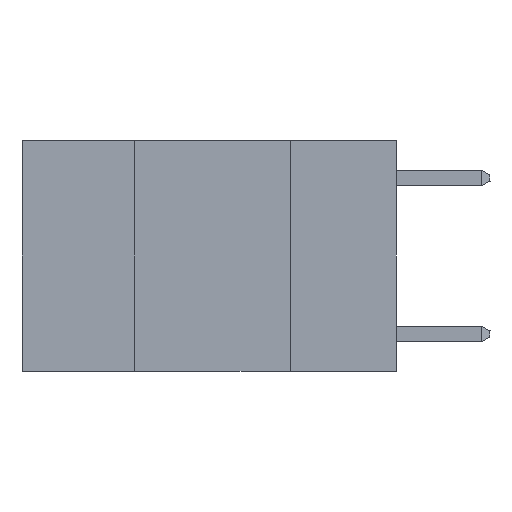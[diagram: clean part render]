
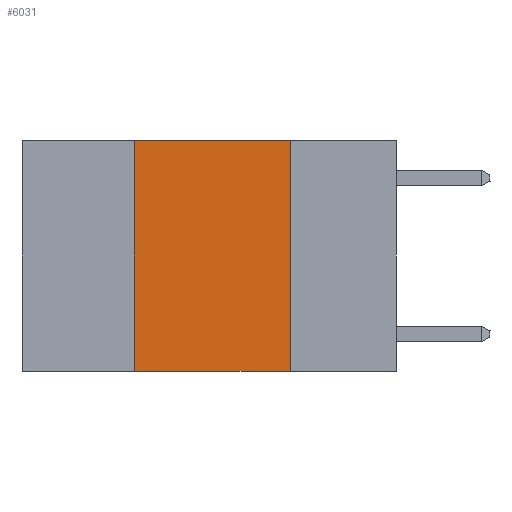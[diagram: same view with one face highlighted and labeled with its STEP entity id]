
A CAD part, left-side view. The second image highlights one B-rep face of the part: STEP entity #6031.
In plain terms, the highlighted planar face has unit normal (-1, 0, 0).
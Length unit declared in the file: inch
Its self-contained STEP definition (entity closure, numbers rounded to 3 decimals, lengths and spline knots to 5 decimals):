
#147 = CARTESIAN_POINT ( 'NONE',  ( 0., 0.6, -0.37 ) ) ;
#323 = LINE ( 'NONE', #3160, #899 ) ;
#630 = VERTEX_POINT ( 'NONE', #1044 ) ;
#771 = VECTOR ( 'NONE', #7086, 39.37008 ) ;
#899 = VECTOR ( 'NONE', #1108, 39.37008 ) ;
#1044 = CARTESIAN_POINT ( 'NONE',  ( 0., 0.17, 0. ) ) ;
#1108 = DIRECTION ( 'NONE',  ( 0., 0., -1. ) ) ;
#1188 = DIRECTION ( 'NONE',  ( 0., 0., -1. ) ) ;
#1454 = CARTESIAN_POINT ( 'NONE',  ( 0., 0.6, 0. ) ) ;
#2038 = LINE ( 'NONE', #6036, #10308 ) ;
#2287 = DIRECTION ( 'NONE',  ( 0., -1., 0. ) ) ;
#2328 = VERTEX_POINT ( 'NONE', #8885 ) ;
#3160 = CARTESIAN_POINT ( 'NONE',  ( 0., 0.17, 0. ) ) ;
#3339 = CARTESIAN_POINT ( 'NONE',  ( 0., 0.42, 0. ) ) ;
#3819 = CARTESIAN_POINT ( 'NONE',  ( 0., 0.6, 0. ) ) ;
#3952 = ORIENTED_EDGE ( 'NONE', *, *, #5118, .F. ) ;
#4251 = DIRECTION ( 'NONE',  ( 1., 0., 0. ) ) ;
#4695 = VECTOR ( 'NONE', #2287, 39.37008 ) ;
#5118 = EDGE_CURVE ( 'NONE', #2328, #12957, #2038, .T. ) ;
#5121 = EDGE_CURVE ( 'NONE', #2328, #10294, #7739, .T. ) ;
#5214 = EDGE_CURVE ( 'NONE', #630, #10294, #323, .T. ) ;
#5470 = PLANE ( 'NONE',  #8064 ) ;
#6031 = ADVANCED_FACE ( 'NONE', ( #10301 ), #5470, .F. ) ;
#6036 = CARTESIAN_POINT ( 'NONE',  ( 0., 0.42, 0. ) ) ;
#6278 = EDGE_LOOP ( 'NONE', ( #6858, #10682, #3952, #12459 ) ) ;
#6858 = ORIENTED_EDGE ( 'NONE', *, *, #5214, .F. ) ;
#7086 = DIRECTION ( 'NONE',  ( 0., -1., 0. ) ) ;
#7739 = LINE ( 'NONE', #147, #4695 ) ;
#8064 = AXIS2_PLACEMENT_3D ( 'NONE', #1454, #4251, #1188 ) ;
#8885 = CARTESIAN_POINT ( 'NONE',  ( 0., 0.42, -0.37 ) ) ;
#9056 = LINE ( 'NONE', #3819, #771 ) ;
#9926 = EDGE_CURVE ( 'NONE', #12957, #630, #9056, .T. ) ;
#10294 = VERTEX_POINT ( 'NONE', #11879 ) ;
#10301 = FACE_OUTER_BOUND ( 'NONE', #6278, .T. ) ;
#10308 = VECTOR ( 'NONE', #10820, 39.37008 ) ;
#10682 = ORIENTED_EDGE ( 'NONE', *, *, #9926, .F. ) ;
#10820 = DIRECTION ( 'NONE',  ( 0., 0., 1. ) ) ;
#11879 = CARTESIAN_POINT ( 'NONE',  ( 0., 0.17, -0.37 ) ) ;
#12459 = ORIENTED_EDGE ( 'NONE', *, *, #5121, .T. ) ;
#12957 = VERTEX_POINT ( 'NONE', #3339 ) ;
